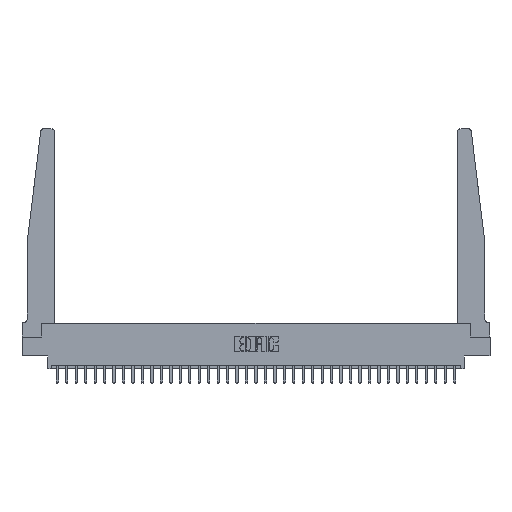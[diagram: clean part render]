
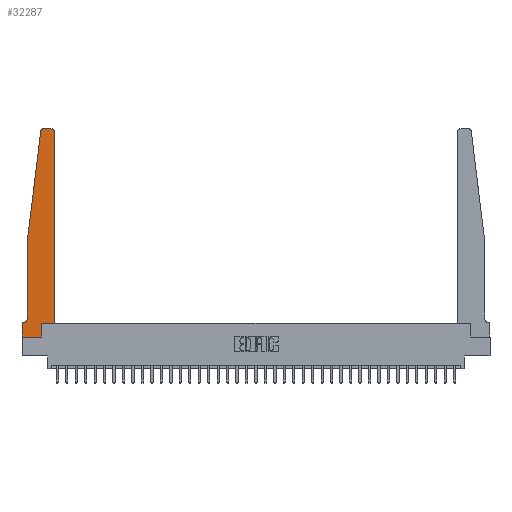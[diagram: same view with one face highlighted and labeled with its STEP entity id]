
A CAD part, top view. The second image highlights one B-rep face of the part: STEP entity #32287.
In plain terms, the highlighted planar face has unit normal (0, 0, 1).
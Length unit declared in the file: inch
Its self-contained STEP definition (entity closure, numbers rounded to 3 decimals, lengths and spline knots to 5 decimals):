
#786 = VERTEX_POINT ( 'NONE', #14901 ) ;
#915 = VERTEX_POINT ( 'NONE', #14653 ) ;
#1054 = VECTOR ( 'NONE', #17343, 39.37008 ) ;
#1439 = ORIENTED_EDGE ( 'NONE', *, *, #10030, .T. ) ;
#1440 = AXIS2_PLACEMENT_3D ( 'NONE', #25160, #6780, #10279 ) ;
#1844 = LINE ( 'NONE', #30263, #14698 ) ;
#1867 = CARTESIAN_POINT ( 'NONE',  ( 0.065, 0.1875, 0.37 ) ) ;
#2347 = DIRECTION ( 'NONE',  ( 1., 0., 0. ) ) ;
#2882 = CARTESIAN_POINT ( 'NONE',  ( 0.425, 0.18, 0.37 ) ) ;
#3043 = ORIENTED_EDGE ( 'NONE', *, *, #10774, .T. ) ;
#3050 = DIRECTION ( 'NONE',  ( -1., 0., 0. ) ) ;
#3576 = DIRECTION ( 'NONE',  ( -1., 0., 0. ) ) ;
#4754 = ORIENTED_EDGE ( 'NONE', *, *, #20703, .T. ) ;
#4932 = EDGE_CURVE ( 'NONE', #786, #29446, #32281, .T. ) ;
#5394 = ORIENTED_EDGE ( 'NONE', *, *, #6303, .T. ) ;
#6102 = EDGE_CURVE ( 'NONE', #7663, #17971, #30123, .T. ) ;
#6247 = LINE ( 'NONE', #16559, #11834 ) ;
#6303 = EDGE_CURVE ( 'NONE', #17141, #32562, #21344, .T. ) ;
#6563 = DIRECTION ( 'NONE',  ( 1., 0., 0. ) ) ;
#6780 = DIRECTION ( 'NONE',  ( 0., 0., 1. ) ) ;
#7103 = PLANE ( 'NONE',  #1440 ) ;
#7438 = ORIENTED_EDGE ( 'NONE', *, *, #32130, .T. ) ;
#7663 = VERTEX_POINT ( 'NONE', #28410 ) ;
#7689 = AXIS2_PLACEMENT_3D ( 'NONE', #11050, #21363, #3576 ) ;
#8043 = VERTEX_POINT ( 'NONE', #30090 ) ;
#8907 = CARTESIAN_POINT ( 'NONE',  ( 0.27653, 2.75, 0.37 ) ) ;
#9075 = DIRECTION ( 'NONE',  ( 0., 0., 1. ) ) ;
#9217 = VERTEX_POINT ( 'NONE', #12534 ) ;
#9406 = VECTOR ( 'NONE', #27198, 39.37008 ) ;
#9432 = CARTESIAN_POINT ( 'NONE',  ( 0., 0., 0.37 ) ) ;
#10030 = EDGE_CURVE ( 'NONE', #27025, #786, #6247, .T. ) ;
#10061 = VECTOR ( 'NONE', #18797, 39.37008 ) ;
#10279 = DIRECTION ( 'NONE',  ( 1., 0., 0. ) ) ;
#10774 = EDGE_CURVE ( 'NONE', #8043, #915, #29254, .T. ) ;
#11050 = CARTESIAN_POINT ( 'NONE',  ( 0.015, 0.2375, 0.37 ) ) ;
#11162 = DIRECTION ( 'NONE',  ( -0.122, -0.992, 0. ) ) ;
#11395 = AXIS2_PLACEMENT_3D ( 'NONE', #29196, #31733, #6563 ) ;
#11628 = CARTESIAN_POINT ( 'NONE',  ( 0.395, 2.72, 0.37 ) ) ;
#11802 = LINE ( 'NONE', #27138, #1054 ) ;
#11811 = EDGE_CURVE ( 'NONE', #29981, #17141, #14149, .T. ) ;
#11834 = VECTOR ( 'NONE', #11162, 39.37008 ) ;
#12534 = CARTESIAN_POINT ( 'NONE',  ( 0.2605, 0., 0.37 ) ) ;
#12693 = VECTOR ( 'NONE', #20161, 39.37008 ) ;
#13091 = CIRCLE ( 'NONE', #7689, 0.05 ) ;
#13158 = CARTESIAN_POINT ( 'NONE',  ( 0.395, 2.75, 0.37 ) ) ;
#14022 = VECTOR ( 'NONE', #16433, 39.37008 ) ;
#14040 = CIRCLE ( 'NONE', #11395, 0.03 ) ;
#14149 = CIRCLE ( 'NONE', #27598, 0.03 ) ;
#14399 = CARTESIAN_POINT ( 'NONE',  ( 0.065, 0.2375, 0.37 ) ) ;
#14653 = CARTESIAN_POINT ( 'NONE',  ( 0.425, 0.18, 0.37 ) ) ;
#14698 = VECTOR ( 'NONE', #2347, 39.37008 ) ;
#14901 = CARTESIAN_POINT ( 'NONE',  ( 0.065, 1.25, 0.37 ) ) ;
#16433 = DIRECTION ( 'NONE',  ( 1., 0., 0. ) ) ;
#16559 = CARTESIAN_POINT ( 'NONE',  ( 0.065, 1.25, 0.37 ) ) ;
#16835 = CARTESIAN_POINT ( 'NONE',  ( 0.425, 2.72, 0.37 ) ) ;
#16849 = DIRECTION ( 'NONE',  ( 1., 0., 0. ) ) ;
#16879 = ORIENTED_EDGE ( 'NONE', *, *, #11811, .T. ) ;
#17026 = EDGE_LOOP ( 'NONE', ( #5394, #4754, #1439, #29550, #21906, #33070, #7438, #27473, #31697, #3043, #32806, #16879 ) ) ;
#17141 = VERTEX_POINT ( 'NONE', #13158 ) ;
#17343 = DIRECTION ( 'NONE',  ( 0., 1., 0. ) ) ;
#17800 = EDGE_CURVE ( 'NONE', #9217, #8043, #11802, .T. ) ;
#17891 = CARTESIAN_POINT ( 'NONE',  ( 0.24675, 2.72367, 0.37 ) ) ;
#17971 = VERTEX_POINT ( 'NONE', #33207 ) ;
#18797 = DIRECTION ( 'NONE',  ( 0., -1., 0. ) ) ;
#18949 = DIRECTION ( 'NONE',  ( 0., 1., 0. ) ) ;
#19120 = CARTESIAN_POINT ( 'NONE',  ( 0.065, 1.25, 0.37 ) ) ;
#19627 = FACE_OUTER_BOUND ( 'NONE', #17026, .T. ) ;
#19757 = EDGE_CURVE ( 'NONE', #29446, #7663, #13091, .T. ) ;
#20161 = DIRECTION ( 'NONE',  ( -1., 0., 0. ) ) ;
#20703 = EDGE_CURVE ( 'NONE', #32562, #27025, #14040, .T. ) ;
#21344 = LINE ( 'NONE', #26213, #22440 ) ;
#21363 = DIRECTION ( 'NONE',  ( 0., 0., -1. ) ) ;
#21510 = EDGE_CURVE ( 'NONE', #915, #29981, #28724, .T. ) ;
#21906 = ORIENTED_EDGE ( 'NONE', *, *, #19757, .T. ) ;
#22015 = LINE ( 'NONE', #31952, #10061 ) ;
#22440 = VECTOR ( 'NONE', #3050, 39.37008 ) ;
#24637 = EDGE_CURVE ( 'NONE', #30772, #9217, #1844, .T. ) ;
#25160 = CARTESIAN_POINT ( 'NONE',  ( 0., 0.1875, 0.37 ) ) ;
#26213 = CARTESIAN_POINT ( 'NONE',  ( 0.25, 2.75, 0.37 ) ) ;
#27025 = VERTEX_POINT ( 'NONE', #17891 ) ;
#27138 = CARTESIAN_POINT ( 'NONE',  ( 0.2605, 0.18, 0.37 ) ) ;
#27198 = DIRECTION ( 'NONE',  ( 0., -1., 0. ) ) ;
#27473 = ORIENTED_EDGE ( 'NONE', *, *, #24637, .T. ) ;
#27598 = AXIS2_PLACEMENT_3D ( 'NONE', #11628, #9075, #16849 ) ;
#28410 = CARTESIAN_POINT ( 'NONE',  ( 0.015, 0.1875, 0.37 ) ) ;
#28724 = LINE ( 'NONE', #31603, #30271 ) ;
#29196 = CARTESIAN_POINT ( 'NONE',  ( 0.27653, 2.72, 0.37 ) ) ;
#29254 = LINE ( 'NONE', #2882, #14022 ) ;
#29446 = VERTEX_POINT ( 'NONE', #14399 ) ;
#29550 = ORIENTED_EDGE ( 'NONE', *, *, #4932, .T. ) ;
#29981 = VERTEX_POINT ( 'NONE', #16835 ) ;
#30090 = CARTESIAN_POINT ( 'NONE',  ( 0.2605, 0.18, 0.37 ) ) ;
#30123 = LINE ( 'NONE', #1867, #12693 ) ;
#30263 = CARTESIAN_POINT ( 'NONE',  ( 0., 0., 0.37 ) ) ;
#30271 = VECTOR ( 'NONE', #18949, 39.37008 ) ;
#30772 = VERTEX_POINT ( 'NONE', #9432 ) ;
#31603 = CARTESIAN_POINT ( 'NONE',  ( 0.425, 0.18, 0.37 ) ) ;
#31697 = ORIENTED_EDGE ( 'NONE', *, *, #17800, .T. ) ;
#31733 = DIRECTION ( 'NONE',  ( 0., 0., 1. ) ) ;
#31952 = CARTESIAN_POINT ( 'NONE',  ( 0., 0., 0.37 ) ) ;
#32130 = EDGE_CURVE ( 'NONE', #17971, #30772, #22015, .T. ) ;
#32281 = LINE ( 'NONE', #19120, #9406 ) ;
#32287 = ADVANCED_FACE ( 'NONE', ( #19627 ), #7103, .T. ) ;
#32562 = VERTEX_POINT ( 'NONE', #8907 ) ;
#32806 = ORIENTED_EDGE ( 'NONE', *, *, #21510, .T. ) ;
#33070 = ORIENTED_EDGE ( 'NONE', *, *, #6102, .T. ) ;
#33207 = CARTESIAN_POINT ( 'NONE',  ( 0., 0.1875, 0.37 ) ) ;
